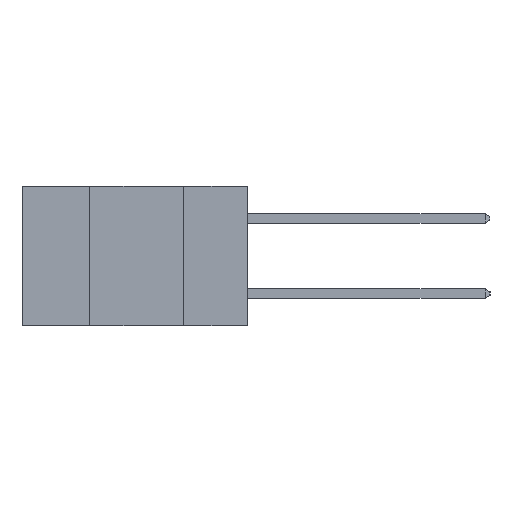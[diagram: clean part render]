
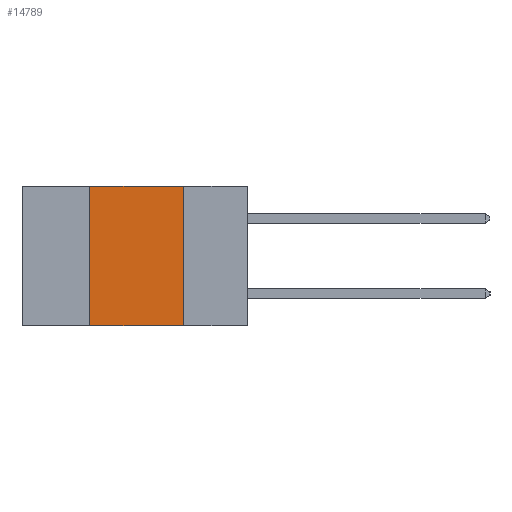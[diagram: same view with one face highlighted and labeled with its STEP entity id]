
A CAD part, left-side view. The second image highlights one B-rep face of the part: STEP entity #14789.
In plain terms, the highlighted planar face has unit normal (-1, 0, 0).
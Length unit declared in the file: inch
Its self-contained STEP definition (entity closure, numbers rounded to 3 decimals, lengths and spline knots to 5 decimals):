
#70 = ORIENTED_EDGE ( 'NONE', *, *, #11818, .F. ) ;
#519 = ORIENTED_EDGE ( 'NONE', *, *, #5053, .F. ) ;
#1794 = PLANE ( 'NONE',  #7273 ) ;
#2685 = VECTOR ( 'NONE', #5017, 39.37008 ) ;
#2963 = CARTESIAN_POINT ( 'NONE',  ( 0., 0.42, -0.37 ) ) ;
#4071 = CARTESIAN_POINT ( 'NONE',  ( 0., 0.6, 0. ) ) ;
#4861 = VERTEX_POINT ( 'NONE', #2963 ) ;
#5017 = DIRECTION ( 'NONE',  ( 0., -1., 0. ) ) ;
#5053 = EDGE_CURVE ( 'NONE', #17509, #14845, #8478, .T. ) ;
#5514 = DIRECTION ( 'NONE',  ( 0., -1., 0. ) ) ;
#5607 = VECTOR ( 'NONE', #11166, 39.37008 ) ;
#5625 = CARTESIAN_POINT ( 'NONE',  ( 0., 0.42, -0.37 ) ) ;
#5741 = EDGE_LOOP ( 'NONE', ( #519, #11304, #70, #10867 ) ) ;
#7073 = DIRECTION ( 'NONE',  ( 0., 0., 1. ) ) ;
#7260 = LINE ( 'NONE', #5625, #17709 ) ;
#7273 = AXIS2_PLACEMENT_3D ( 'NONE', #15743, #7532, #17072 ) ;
#7532 = DIRECTION ( 'NONE',  ( 1., 0., 0. ) ) ;
#8478 = LINE ( 'NONE', #9174, #5607 ) ;
#9124 = FACE_OUTER_BOUND ( 'NONE', #5741, .T. ) ;
#9174 = CARTESIAN_POINT ( 'NONE',  ( 0., 0.17, -0.37 ) ) ;
#9281 = CARTESIAN_POINT ( 'NONE',  ( 0., 0.6, -0.37 ) ) ;
#10867 = ORIENTED_EDGE ( 'NONE', *, *, #14961, .T. ) ;
#11047 = EDGE_CURVE ( 'NONE', #15674, #17509, #12047, .T. ) ;
#11166 = DIRECTION ( 'NONE',  ( 0., 0., -1. ) ) ;
#11304 = ORIENTED_EDGE ( 'NONE', *, *, #11047, .F. ) ;
#11623 = VECTOR ( 'NONE', #5514, 39.37008 ) ;
#11818 = EDGE_CURVE ( 'NONE', #4861, #15674, #7260, .T. ) ;
#12047 = LINE ( 'NONE', #4071, #11623 ) ;
#12497 = CARTESIAN_POINT ( 'NONE',  ( 0., 0.42, 0. ) ) ;
#12563 = CARTESIAN_POINT ( 'NONE',  ( 0., 0.17, 0. ) ) ;
#13135 = CARTESIAN_POINT ( 'NONE',  ( 0., 0.17, -0.37 ) ) ;
#14789 = ADVANCED_FACE ( 'NONE', ( #9124 ), #1794, .F. ) ;
#14845 = VERTEX_POINT ( 'NONE', #13135 ) ;
#14961 = EDGE_CURVE ( 'NONE', #4861, #14845, #16997, .T. ) ;
#15674 = VERTEX_POINT ( 'NONE', #12497 ) ;
#15743 = CARTESIAN_POINT ( 'NONE',  ( 0., 0.6, 0. ) ) ;
#16997 = LINE ( 'NONE', #9281, #2685 ) ;
#17072 = DIRECTION ( 'NONE',  ( 0., 0., -1. ) ) ;
#17509 = VERTEX_POINT ( 'NONE', #12563 ) ;
#17709 = VECTOR ( 'NONE', #7073, 39.37008 ) ;
